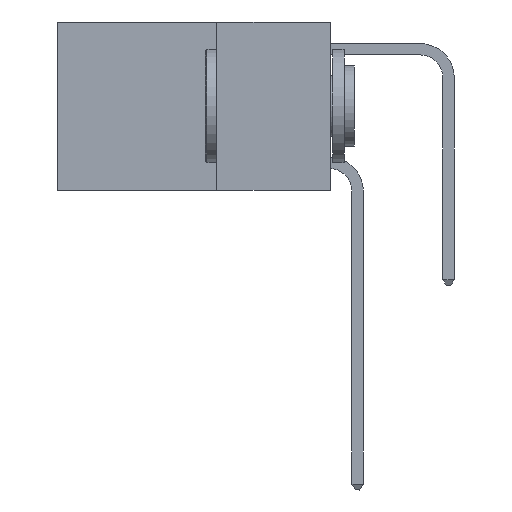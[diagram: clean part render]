
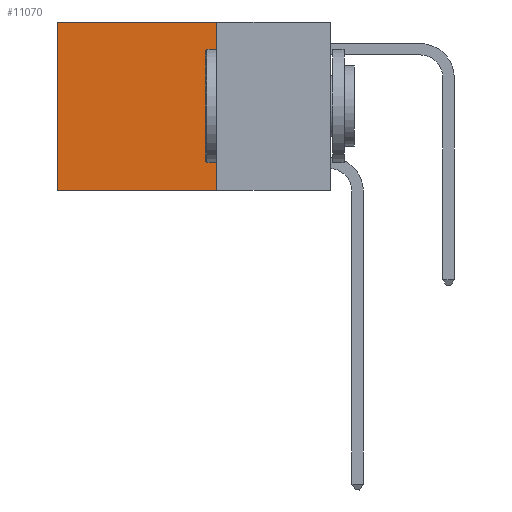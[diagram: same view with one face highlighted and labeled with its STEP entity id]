
A CAD part, left-side view. The second image highlights one B-rep face of the part: STEP entity #11070.
In plain terms, the highlighted planar face has unit normal (-1, 0, 0).
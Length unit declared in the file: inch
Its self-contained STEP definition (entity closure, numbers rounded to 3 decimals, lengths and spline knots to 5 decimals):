
#55 = CARTESIAN_POINT ( 'NONE',  ( 0.2625, 0.25, -0.37 ) ) ;
#756 = CARTESIAN_POINT ( 'NONE',  ( 0.2625, 0.25, 0. ) ) ;
#2211 = LINE ( 'NONE', #17339, #18570 ) ;
#2394 = CARTESIAN_POINT ( 'NONE',  ( 0.2625, 0.25, 0. ) ) ;
#3132 = DIRECTION ( 'NONE',  ( 0., 1., 0. ) ) ;
#3274 = EDGE_CURVE ( 'NONE', #9217, #9760, #11440, .T. ) ;
#5757 = CARTESIAN_POINT ( 'NONE',  ( 0.2625, 0.6, -0.37 ) ) ;
#7558 = ORIENTED_EDGE ( 'NONE', *, *, #15426, .T. ) ;
#8868 = DIRECTION ( 'NONE',  ( 1., 0., 0. ) ) ;
#9217 = VERTEX_POINT ( 'NONE', #13693 ) ;
#9291 = AXIS2_PLACEMENT_3D ( 'NONE', #756, #8868, #19822 ) ;
#9760 = VERTEX_POINT ( 'NONE', #5757 ) ;
#9802 = DIRECTION ( 'NONE',  ( 0., 0., -1. ) ) ;
#10023 = ORIENTED_EDGE ( 'NONE', *, *, #3274, .T. ) ;
#10081 = ORIENTED_EDGE ( 'NONE', *, *, #16605, .F. ) ;
#10100 = ORIENTED_EDGE ( 'NONE', *, *, #17967, .F. ) ;
#11028 = LINE ( 'NONE', #11399, #18846 ) ;
#11070 = ADVANCED_FACE ( 'NONE', ( #18832 ), #15150, .F. ) ;
#11399 = CARTESIAN_POINT ( 'NONE',  ( 0.2625, 0.25, 0. ) ) ;
#11440 = LINE ( 'NONE', #13951, #19247 ) ;
#12968 = EDGE_LOOP ( 'NONE', ( #10023, #10100, #10081, #7558 ) ) ;
#13693 = CARTESIAN_POINT ( 'NONE',  ( 0.2625, 0.6, 0. ) ) ;
#13951 = CARTESIAN_POINT ( 'NONE',  ( 0.2625, 0.6, 0. ) ) ;
#14254 = VECTOR ( 'NONE', #18068, 39.37008 ) ;
#15150 = PLANE ( 'NONE',  #9291 ) ;
#15426 = EDGE_CURVE ( 'NONE', #18901, #9217, #18416, .T. ) ;
#15530 = DIRECTION ( 'NONE',  ( 0., 0., -1. ) ) ;
#16490 = CARTESIAN_POINT ( 'NONE',  ( 0.2625, 0.25, 0. ) ) ;
#16605 = EDGE_CURVE ( 'NONE', #18901, #18082, #11028, .T. ) ;
#17339 = CARTESIAN_POINT ( 'NONE',  ( 0.2625, 0.25, -0.37 ) ) ;
#17967 = EDGE_CURVE ( 'NONE', #18082, #9760, #2211, .T. ) ;
#18068 = DIRECTION ( 'NONE',  ( 0., 1., 0. ) ) ;
#18082 = VERTEX_POINT ( 'NONE', #55 ) ;
#18416 = LINE ( 'NONE', #16490, #14254 ) ;
#18570 = VECTOR ( 'NONE', #3132, 39.37008 ) ;
#18832 = FACE_OUTER_BOUND ( 'NONE', #12968, .T. ) ;
#18846 = VECTOR ( 'NONE', #9802, 39.37008 ) ;
#18901 = VERTEX_POINT ( 'NONE', #2394 ) ;
#19247 = VECTOR ( 'NONE', #15530, 39.37008 ) ;
#19822 = DIRECTION ( 'NONE',  ( 0., 0., -1. ) ) ;
